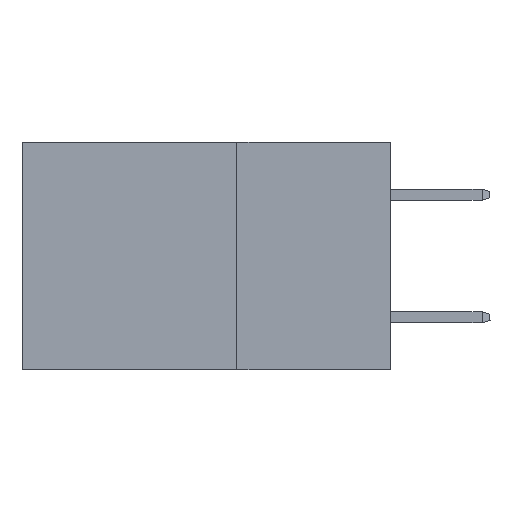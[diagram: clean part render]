
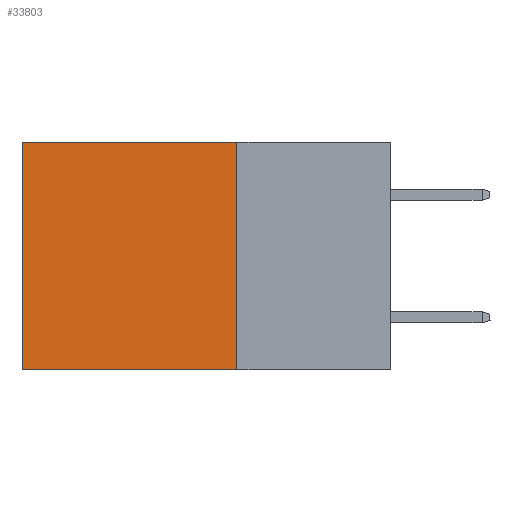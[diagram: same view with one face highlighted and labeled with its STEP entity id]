
A CAD part, left-side view. The second image highlights one B-rep face of the part: STEP entity #33803.
In plain terms, the highlighted planar face has unit normal (-1, 0, 0).
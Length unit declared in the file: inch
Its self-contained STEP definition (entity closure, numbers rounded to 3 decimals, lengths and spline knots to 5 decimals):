
#2814 = VECTOR ( 'NONE', #10010, 39.37008 ) ;
#3610 = EDGE_LOOP ( 'NONE', ( #13510, #26209, #19209, #20615 ) ) ;
#6227 = DIRECTION ( 'NONE',  ( 0., 0., -1. ) ) ;
#8146 = DIRECTION ( 'NONE',  ( 0., 1., 0. ) ) ;
#9378 = FACE_OUTER_BOUND ( 'NONE', #3610, .T. ) ;
#10010 = DIRECTION ( 'NONE',  ( 0., 1., 0. ) ) ;
#10052 = DIRECTION ( 'NONE',  ( 0., 0., -1. ) ) ;
#12996 = CARTESIAN_POINT ( 'NONE',  ( 0.2875, 0.6, 0. ) ) ;
#13510 = ORIENTED_EDGE ( 'NONE', *, *, #39409, .T. ) ;
#13531 = PLANE ( 'NONE',  #38071 ) ;
#17022 = CARTESIAN_POINT ( 'NONE',  ( 0.2875, 0.25, 0. ) ) ;
#18202 = CARTESIAN_POINT ( 'NONE',  ( 0.2875, 0.25, 0. ) ) ;
#18645 = VECTOR ( 'NONE', #21696, 39.37008 ) ;
#19209 = ORIENTED_EDGE ( 'NONE', *, *, #45172, .F. ) ;
#19492 = CARTESIAN_POINT ( 'NONE',  ( 0.2875, 0.25, -0.37 ) ) ;
#19866 = VERTEX_POINT ( 'NONE', #12996 ) ;
#20615 = ORIENTED_EDGE ( 'NONE', *, *, #31243, .T. ) ;
#21565 = EDGE_CURVE ( 'NONE', #28323, #31248, #43641, .T. ) ;
#21696 = DIRECTION ( 'NONE',  ( 0., 0., -1. ) ) ;
#24167 = CARTESIAN_POINT ( 'NONE',  ( 0.2875, 0.6, -0.37 ) ) ;
#24439 = DIRECTION ( 'NONE',  ( 1., 0., 0. ) ) ;
#24828 = VERTEX_POINT ( 'NONE', #42817 ) ;
#25421 = LINE ( 'NONE', #18202, #18645 ) ;
#26209 = ORIENTED_EDGE ( 'NONE', *, *, #21565, .F. ) ;
#27149 = CARTESIAN_POINT ( 'NONE',  ( 0.2875, 0.6, 0. ) ) ;
#28323 = VERTEX_POINT ( 'NONE', #29388 ) ;
#29388 = CARTESIAN_POINT ( 'NONE',  ( 0.2875, 0.25, -0.37 ) ) ;
#31243 = EDGE_CURVE ( 'NONE', #24828, #19866, #41787, .T. ) ;
#31248 = VERTEX_POINT ( 'NONE', #24167 ) ;
#32477 = VECTOR ( 'NONE', #6227, 39.37008 ) ;
#33803 = ADVANCED_FACE ( 'NONE', ( #9378 ), #13531, .F. ) ;
#35862 = VECTOR ( 'NONE', #8146, 39.37008 ) ;
#37863 = CARTESIAN_POINT ( 'NONE',  ( 0.2875, 0.25, 0. ) ) ;
#38071 = AXIS2_PLACEMENT_3D ( 'NONE', #17022, #24439, #10052 ) ;
#39409 = EDGE_CURVE ( 'NONE', #19866, #31248, #40829, .T. ) ;
#40829 = LINE ( 'NONE', #27149, #32477 ) ;
#41787 = LINE ( 'NONE', #37863, #2814 ) ;
#42817 = CARTESIAN_POINT ( 'NONE',  ( 0.2875, 0.25, 0. ) ) ;
#43641 = LINE ( 'NONE', #19492, #35862 ) ;
#45172 = EDGE_CURVE ( 'NONE', #24828, #28323, #25421, .T. ) ;
